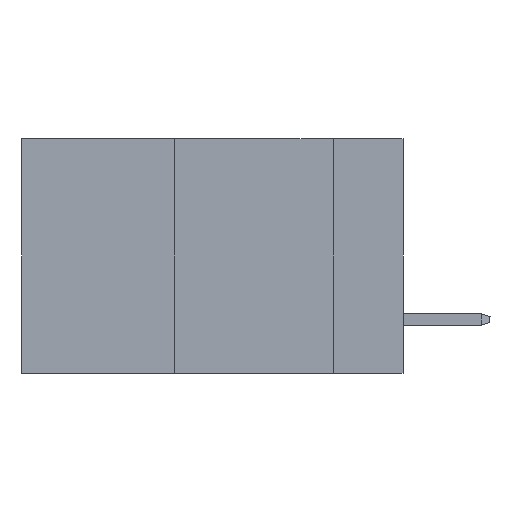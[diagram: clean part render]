
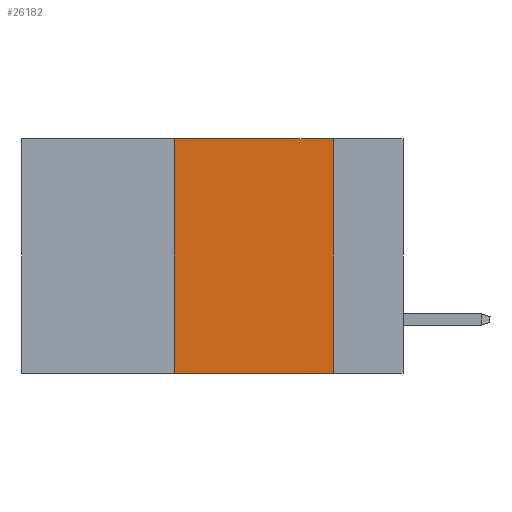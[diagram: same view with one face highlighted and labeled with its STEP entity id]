
A CAD part, left-side view. The second image highlights one B-rep face of the part: STEP entity #26182.
In plain terms, the highlighted planar face has unit normal (-1, 0, 0).
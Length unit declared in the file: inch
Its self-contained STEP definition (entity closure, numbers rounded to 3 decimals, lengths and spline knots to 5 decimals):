
#156 = ORIENTED_EDGE ( 'NONE', *, *, #9282, .F. ) ;
#594 = EDGE_CURVE ( 'NONE', #26077, #8109, #3857, .T. ) ;
#1047 = DIRECTION ( 'NONE',  ( 0., 0., -1. ) ) ;
#2750 = LINE ( 'NONE', #11007, #19082 ) ;
#2916 = ORIENTED_EDGE ( 'NONE', *, *, #594, .F. ) ;
#3460 = EDGE_CURVE ( 'NONE', #6791, #9782, #2750, .T. ) ;
#3857 = LINE ( 'NONE', #20411, #13375 ) ;
#5104 = LINE ( 'NONE', #25609, #16996 ) ;
#5244 = DIRECTION ( 'NONE',  ( 0., 0., 1. ) ) ;
#5288 = LINE ( 'NONE', #13562, #19300 ) ;
#6297 = ORIENTED_EDGE ( 'NONE', *, *, #7930, .F. ) ;
#6607 = ORIENTED_EDGE ( 'NONE', *, *, #3460, .T. ) ;
#6791 = VERTEX_POINT ( 'NONE', #17080 ) ;
#7930 = EDGE_CURVE ( 'NONE', #6791, #26077, #5104, .T. ) ;
#8109 = VERTEX_POINT ( 'NONE', #18282 ) ;
#9282 = EDGE_CURVE ( 'NONE', #8109, #9782, #5288, .T. ) ;
#9459 = DIRECTION ( 'NONE',  ( 1., 0., 0. ) ) ;
#9759 = DIRECTION ( 'NONE',  ( 0., 0., -1. ) ) ;
#9782 = VERTEX_POINT ( 'NONE', #24625 ) ;
#10095 = DIRECTION ( 'NONE',  ( 0., -1., 0. ) ) ;
#11007 = CARTESIAN_POINT ( 'NONE',  ( 0., 0.6, -0.37 ) ) ;
#11496 = CARTESIAN_POINT ( 'NONE',  ( 0., 0.6, 0. ) ) ;
#13375 = VECTOR ( 'NONE', #10095, 39.37008 ) ;
#13562 = CARTESIAN_POINT ( 'NONE',  ( 0., 0.11, 0. ) ) ;
#15998 = AXIS2_PLACEMENT_3D ( 'NONE', #11496, #9459, #1047 ) ;
#16996 = VECTOR ( 'NONE', #5244, 39.37008 ) ;
#17080 = CARTESIAN_POINT ( 'NONE',  ( 0., 0.36, -0.37 ) ) ;
#18282 = CARTESIAN_POINT ( 'NONE',  ( 0., 0.11, 0. ) ) ;
#19082 = VECTOR ( 'NONE', #19305, 39.37008 ) ;
#19300 = VECTOR ( 'NONE', #9759, 39.37008 ) ;
#19305 = DIRECTION ( 'NONE',  ( 0., -1., 0. ) ) ;
#20069 = FACE_OUTER_BOUND ( 'NONE', #21497, .T. ) ;
#20411 = CARTESIAN_POINT ( 'NONE',  ( 0., 0.6, 0. ) ) ;
#21497 = EDGE_LOOP ( 'NONE', ( #156, #2916, #6297, #6607 ) ) ;
#23583 = CARTESIAN_POINT ( 'NONE',  ( 0., 0.36, 0. ) ) ;
#24129 = PLANE ( 'NONE',  #15998 ) ;
#24625 = CARTESIAN_POINT ( 'NONE',  ( 0., 0.11, -0.37 ) ) ;
#25609 = CARTESIAN_POINT ( 'NONE',  ( 0., 0.36, 0. ) ) ;
#26077 = VERTEX_POINT ( 'NONE', #23583 ) ;
#26182 = ADVANCED_FACE ( 'NONE', ( #20069 ), #24129, .F. ) ;
